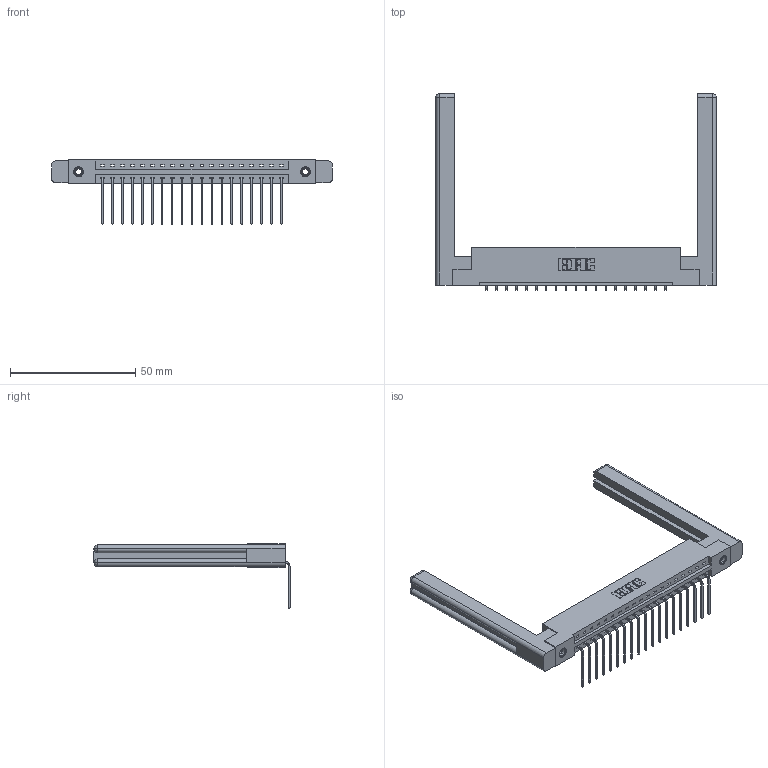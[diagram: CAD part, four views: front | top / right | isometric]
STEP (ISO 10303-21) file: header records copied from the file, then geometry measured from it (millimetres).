
FILE_DESCRIPTION (( 'STEP AP203' ), '1' );
FILE_NAME ('387-019-559-158.STEP', '2019-10-02T21:55:52', ( '' ), ( '' ), 'SwSTEP 2.0', 'SolidWorks 2016', '' );
FILE_SCHEMA (( 'CONFIG_CONTROL_DESIGN' ));
Length unit declared in the file: inch
Products named in the file (5): 345-292-001_558 559 Tail - 1; 345-250-001_345-250-001-102; 387-019-559-158; 307-220-058; 337 Part_Flush Mounting Lugs - 0.156 Dia-TI
Assembly tree (24 placements, depth 2):
  387-019-559-158
    337 Part_Flush Mounting Lugs - 0.156 Dia-TI
    345-292-001_558 559 Tail - 1  x19
    345-250-001_345-250-001-102  x2
    307-220-058  x2
Bounding box: 111.91 x 78.17 x 25.53 mm (x, y, z)
Volume: 18569.1 mm3; surface area: 17261.6 mm2
Topology: 24 solids, 24 shells, 1472 faces, 4351 edges, 2862 vertices
Faces by surface type: plane 1066, cylinder 382, cone 12, torus 12
Entity records: 19816 total; most frequent: CARTESIAN_POINT 3450, ORIENTED_EDGE 3344, DIRECTION 2970, EDGE_CURVE 1672, LINE 1496, VECTOR 1496, VERTEX_POINT 1106, AXIS2_PLACEMENT_3D 737
